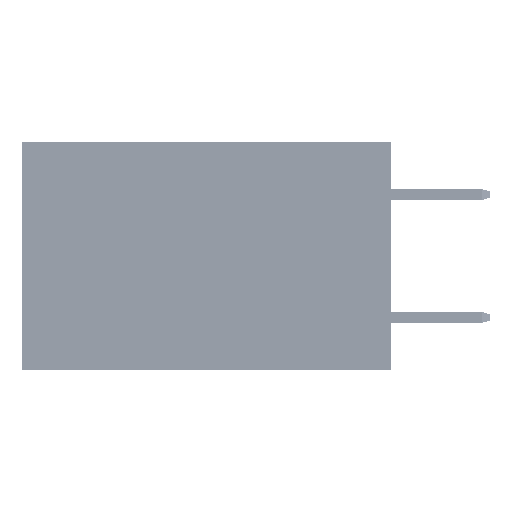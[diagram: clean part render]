
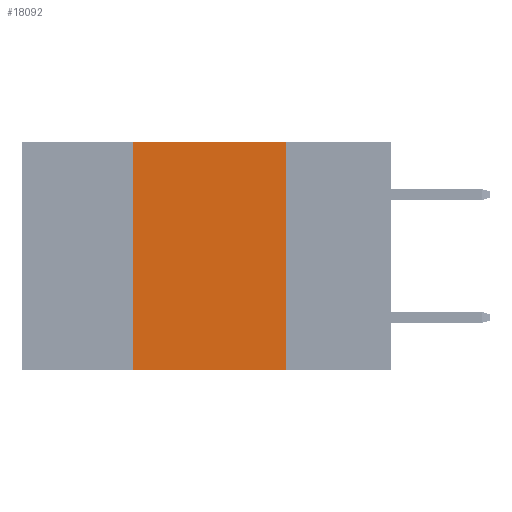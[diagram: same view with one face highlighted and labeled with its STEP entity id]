
A CAD part, left-side view. The second image highlights one B-rep face of the part: STEP entity #18092.
In plain terms, the highlighted planar face has unit normal (-1, 0, 0).
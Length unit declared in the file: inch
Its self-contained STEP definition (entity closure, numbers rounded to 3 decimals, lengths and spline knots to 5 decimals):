
#731 = CARTESIAN_POINT ( 'NONE',  ( 0., 0.42, -0.37 ) ) ;
#1542 = ORIENTED_EDGE ( 'NONE', *, *, #32959, .F. ) ;
#3396 = DIRECTION ( 'NONE',  ( 0., 0., -1. ) ) ;
#3722 = EDGE_CURVE ( 'NONE', #16646, #34513, #10103, .T. ) ;
#5661 = VERTEX_POINT ( 'NONE', #40636 ) ;
#6446 = VECTOR ( 'NONE', #27827, 39.37008 ) ;
#6767 = LINE ( 'NONE', #23125, #16125 ) ;
#8913 = DIRECTION ( 'NONE',  ( 0., 0., -1. ) ) ;
#10103 = LINE ( 'NONE', #36676, #40464 ) ;
#12720 = EDGE_CURVE ( 'NONE', #32585, #5661, #28884, .T. ) ;
#14349 = AXIS2_PLACEMENT_3D ( 'NONE', #46883, #15262, #3396 ) ;
#15262 = DIRECTION ( 'NONE',  ( 1., 0., 0. ) ) ;
#16125 = VECTOR ( 'NONE', #23301, 39.37008 ) ;
#16646 = VERTEX_POINT ( 'NONE', #18549 ) ;
#18092 = ADVANCED_FACE ( 'NONE', ( #44818 ), #50799, .F. ) ;
#18549 = CARTESIAN_POINT ( 'NONE',  ( 0., 0.17, 0. ) ) ;
#19282 = ORIENTED_EDGE ( 'NONE', *, *, #3722, .F. ) ;
#23125 = CARTESIAN_POINT ( 'NONE',  ( 0., 0.6, -0.37 ) ) ;
#23301 = DIRECTION ( 'NONE',  ( 0., -1., 0. ) ) ;
#23878 = VECTOR ( 'NONE', #46090, 39.37008 ) ;
#27827 = DIRECTION ( 'NONE',  ( 0., 0., 1. ) ) ;
#28884 = LINE ( 'NONE', #47446, #6446 ) ;
#29713 = EDGE_CURVE ( 'NONE', #32585, #34513, #6767, .T. ) ;
#32585 = VERTEX_POINT ( 'NONE', #731 ) ;
#32959 = EDGE_CURVE ( 'NONE', #5661, #16646, #33168, .T. ) ;
#33168 = LINE ( 'NONE', #38349, #23878 ) ;
#34513 = VERTEX_POINT ( 'NONE', #39762 ) ;
#36676 = CARTESIAN_POINT ( 'NONE',  ( 0., 0.17, 0. ) ) ;
#37075 = ORIENTED_EDGE ( 'NONE', *, *, #12720, .F. ) ;
#38349 = CARTESIAN_POINT ( 'NONE',  ( 0., 0.6, 0. ) ) ;
#39762 = CARTESIAN_POINT ( 'NONE',  ( 0., 0.17, -0.37 ) ) ;
#39888 = EDGE_LOOP ( 'NONE', ( #19282, #1542, #37075, #46609 ) ) ;
#40464 = VECTOR ( 'NONE', #8913, 39.37008 ) ;
#40636 = CARTESIAN_POINT ( 'NONE',  ( 0., 0.42, 0. ) ) ;
#44818 = FACE_OUTER_BOUND ( 'NONE', #39888, .T. ) ;
#46090 = DIRECTION ( 'NONE',  ( 0., -1., 0. ) ) ;
#46609 = ORIENTED_EDGE ( 'NONE', *, *, #29713, .T. ) ;
#46883 = CARTESIAN_POINT ( 'NONE',  ( 0., 0.6, 0. ) ) ;
#47446 = CARTESIAN_POINT ( 'NONE',  ( 0., 0.42, 0. ) ) ;
#50799 = PLANE ( 'NONE',  #14349 ) ;
